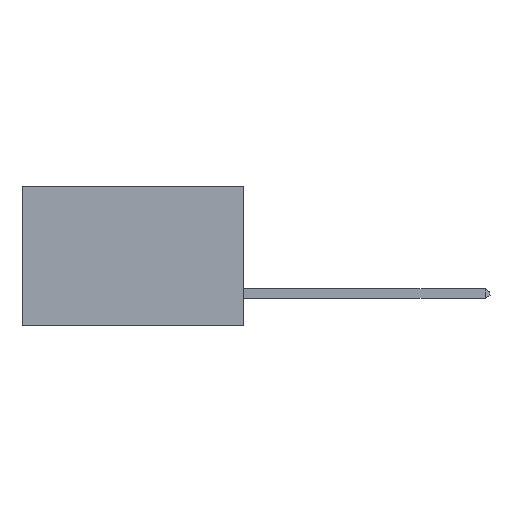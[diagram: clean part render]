
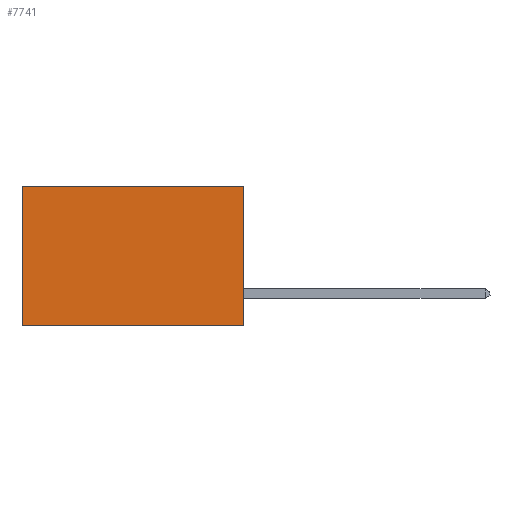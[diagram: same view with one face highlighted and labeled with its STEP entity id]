
A CAD part, left-side view. The second image highlights one B-rep face of the part: STEP entity #7741.
In plain terms, the highlighted planar face has unit normal (-1, 0, 0).
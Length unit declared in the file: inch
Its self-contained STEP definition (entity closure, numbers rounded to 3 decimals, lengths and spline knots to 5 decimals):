
#135 = VERTEX_POINT ( 'NONE', #7443 ) ;
#140 = DIRECTION ( 'NONE',  ( 0., 0., -1. ) ) ;
#188 = CARTESIAN_POINT ( 'NONE',  ( 0.277, 0., 0. ) ) ;
#499 = AXIS2_PLACEMENT_3D ( 'NONE', #8661, #9504, #4335 ) ;
#943 = FACE_OUTER_BOUND ( 'NONE', #8591, .T. ) ;
#1518 = EDGE_CURVE ( 'NONE', #3445, #6385, #8881, .T. ) ;
#1571 = CARTESIAN_POINT ( 'NONE',  ( 0.277, 0.59, 0. ) ) ;
#1825 = CARTESIAN_POINT ( 'NONE',  ( 0.277, 0., -0.37 ) ) ;
#3445 = VERTEX_POINT ( 'NONE', #1825 ) ;
#3637 = DIRECTION ( 'NONE',  ( 0., 0., -1. ) ) ;
#4335 = DIRECTION ( 'NONE',  ( 0., 0., -1. ) ) ;
#4677 = CARTESIAN_POINT ( 'NONE',  ( 0.277, 0., -0.37 ) ) ;
#5568 = ORIENTED_EDGE ( 'NONE', *, *, #1518, .F. ) ;
#5595 = LINE ( 'NONE', #8878, #10133 ) ;
#5953 = VECTOR ( 'NONE', #140, 39.37008 ) ;
#6385 = VERTEX_POINT ( 'NONE', #7716 ) ;
#6461 = VERTEX_POINT ( 'NONE', #1571 ) ;
#6524 = VECTOR ( 'NONE', #10683, 39.37008 ) ;
#6611 = VECTOR ( 'NONE', #8398, 39.37008 ) ;
#7339 = ORIENTED_EDGE ( 'NONE', *, *, #10159, .T. ) ;
#7443 = CARTESIAN_POINT ( 'NONE',  ( 0.277, 0., 0. ) ) ;
#7716 = CARTESIAN_POINT ( 'NONE',  ( 0.277, 0.59, -0.37 ) ) ;
#7741 = ADVANCED_FACE ( 'NONE', ( #943 ), #7829, .F. ) ;
#7829 = PLANE ( 'NONE',  #499 ) ;
#8005 = EDGE_CURVE ( 'NONE', #135, #6461, #8791, .T. ) ;
#8398 = DIRECTION ( 'NONE',  ( 0., 1., 0. ) ) ;
#8458 = EDGE_CURVE ( 'NONE', #135, #3445, #10999, .T. ) ;
#8591 = EDGE_LOOP ( 'NONE', ( #7339, #5568, #9436, #10752 ) ) ;
#8661 = CARTESIAN_POINT ( 'NONE',  ( 0.277, 0., -0.37 ) ) ;
#8791 = LINE ( 'NONE', #188, #6524 ) ;
#8878 = CARTESIAN_POINT ( 'NONE',  ( 0.277, 0.59, -0.37 ) ) ;
#8881 = LINE ( 'NONE', #4677, #6611 ) ;
#9436 = ORIENTED_EDGE ( 'NONE', *, *, #8458, .F. ) ;
#9504 = DIRECTION ( 'NONE',  ( 1., 0., 0. ) ) ;
#10133 = VECTOR ( 'NONE', #3637, 39.37008 ) ;
#10159 = EDGE_CURVE ( 'NONE', #6461, #6385, #5595, .T. ) ;
#10636 = CARTESIAN_POINT ( 'NONE',  ( 0.277, 0., -0.37 ) ) ;
#10683 = DIRECTION ( 'NONE',  ( 0., 1., 0. ) ) ;
#10752 = ORIENTED_EDGE ( 'NONE', *, *, #8005, .T. ) ;
#10999 = LINE ( 'NONE', #10636, #5953 ) ;
